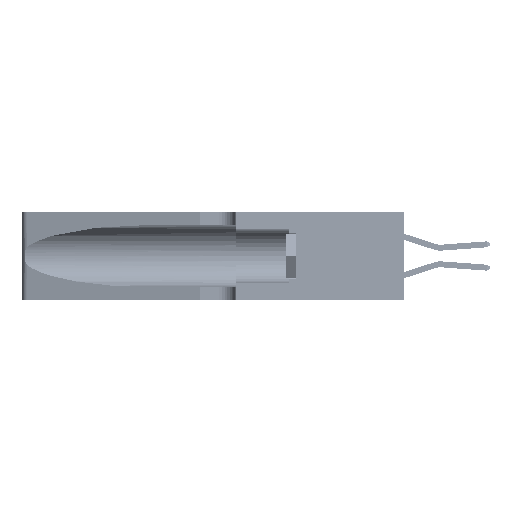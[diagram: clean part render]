
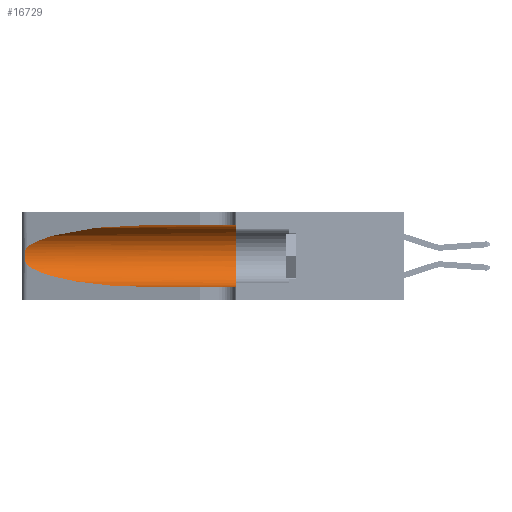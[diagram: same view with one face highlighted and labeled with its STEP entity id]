
A CAD part, left-side view. The second image highlights one B-rep face of the part: STEP entity #16729.
In plain terms, the highlighted cylindrical face has radius 3.308 mm (diameter 6.617 mm), a partial arc.
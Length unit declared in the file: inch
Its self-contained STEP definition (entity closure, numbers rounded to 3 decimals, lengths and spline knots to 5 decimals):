
#296 = CARTESIAN_POINT ( 'NONE',  ( 0.25854, 1.2359, 0.20912 ) ) ;
#1487 = DIRECTION ( 'NONE',  ( 0., -1., 0. ) ) ;
#2696 = FACE_OUTER_BOUND ( 'NONE', #32407, .T. ) ;
#2927 = CARTESIAN_POINT ( 'NONE',  ( 0.1305, 1.61858, 0.185 ) ) ;
#4195 = CARTESIAN_POINT ( 'NONE',  ( 0.1305, 0.35, 0.05475 ) ) ;
#4247 = VECTOR ( 'NONE', #1487, 39.37008 ) ;
#4519 = CARTESIAN_POINT ( 'NONE',  ( 0.25639, 1.23184, 0.21858 ) ) ;
#4634 = CARTESIAN_POINT ( 'NONE',  ( 0.1305, 0.72297, 0.31525 ) ) ;
#5460 = ORIENTED_EDGE ( 'NONE', *, *, #12467, .T. ) ;
#7127 = CARTESIAN_POINT ( 'NONE',  ( 0.25487, 1.22718, 0.14631 ) ) ;
#7469 = CARTESIAN_POINT ( 'NONE',  ( 0.18966, 0.96281, 0.05475 ) ) ;
#8483 = CARTESIAN_POINT ( 'NONE',  ( 0.26075, 1.23896, 0.19203 ) ) ;
#8582 = EDGE_CURVE ( 'NONE', #26187, #10819, #14224, .T. ) ;
#9706 = CARTESIAN_POINT ( 'NONE',  ( 0.25639, 1.23186, 0.15144 ) ) ;
#10405 = CARTESIAN_POINT ( 'NONE',  ( 0.25789, 1.23486, 0.15765 ) ) ;
#10819 = VERTEX_POINT ( 'NONE', #4195 ) ;
#11353 = VERTEX_POINT ( 'NONE', #22461 ) ;
#11595 = DIRECTION ( 'NONE',  ( 0., -1., 0. ) ) ;
#12467 = EDGE_CURVE ( 'NONE', #36347, #12877, #46049, .T. ) ;
#12497 = VERTEX_POINT ( 'NONE', #17984 ) ;
#12662 = CARTESIAN_POINT ( 'NONE',  ( 0.25555, 1.22994, 0.2215 ) ) ;
#12877 = VERTEX_POINT ( 'NONE', #31217 ) ;
#13211 = ORIENTED_EDGE ( 'NONE', *, *, #38663, .T. ) ;
#13757 = EDGE_CURVE ( 'NONE', #12877, #11353, #20491, .T. ) ;
#14224 = LINE ( 'NONE', #40901, #4247 ) ;
#16729 = ADVANCED_FACE ( 'NONE', ( #2696 ), #19548, .F. ) ;
#16826 = CARTESIAN_POINT ( 'NONE',  ( 0.25487, 1.22718, 0.22369 ) ) ;
#17875 = CARTESIAN_POINT ( 'NONE',  ( 0.26075, 1.23896, 0.178 ) ) ;
#17984 = CARTESIAN_POINT ( 'NONE',  ( 0.1305, 0.35, 0.31525 ) ) ;
#19548 = CYLINDRICAL_SURFACE ( 'NONE', #30772, 0.13025 ) ;
#19705 = ORIENTED_EDGE ( 'NONE', *, *, #23955, .F. ) ;
#20341 = CARTESIAN_POINT ( 'NONE',  ( 0.25787, 1.23484, 0.2124 ) ) ;
#20491 = B_SPLINE_CURVE_WITH_KNOTS ( 'NONE', 3,
 ( #16826, #12662, #4519, #20341, #296, #28178, #8483, #17875, #34284, #22074, #10405, #9706, #37609, #45628 ),
 .UNSPECIFIED., .F., .F.,
 ( 4, 2, 2, 2, 2, 2, 4 ),
 ( 0., 0.00027, 0.00053, 0.00107, 0.0016, 0.00187, 0.00214 ),
 .UNSPECIFIED. ) ;
#20998 = ORIENTED_EDGE ( 'NONE', *, *, #13757, .T. ) ;
#22074 = CARTESIAN_POINT ( 'NONE',  ( 0.25856, 1.23593, 0.16098 ) ) ;
#22461 = CARTESIAN_POINT ( 'NONE',  ( 0.25487, 1.22718, 0.14631 ) ) ;
#23955 = EDGE_CURVE ( 'NONE', #36347, #12497, #46667, .T. ) ;
#24228 = DIRECTION ( 'NONE',  ( 0., 1., 0. ) ) ;
#26187 = VERTEX_POINT ( 'NONE', #33351 ) ;
#26600 = DIRECTION ( 'NONE',  ( 0., 0., -1. ) ) ;
#27503 = CARTESIAN_POINT ( 'NONE',  ( 0.1305, 0.72297, 0.05475 ) ) ;
#28178 = CARTESIAN_POINT ( 'NONE',  ( 0.26018, 1.23835, 0.19895 ) ) ;
#29765 =( BOUNDED_CURVE ( )  B_SPLINE_CURVE ( 3, ( #7127, #38864, #7469, #27503 ),
 .UNSPECIFIED., .F., .T. ) 
 B_SPLINE_CURVE_WITH_KNOTS ( ( 4, 4 ),
 ( 3.44316, 4.71239 ),
 .UNSPECIFIED. ) 
 CURVE ( )  GEOMETRIC_REPRESENTATION_ITEM ( )  RATIONAL_B_SPLINE_CURVE ( ( 1., 0.87, 0.87, 1. ) ) 
 REPRESENTATION_ITEM ( '' )  );
#30772 = AXIS2_PLACEMENT_3D ( 'NONE', #2927, #34487, #26600 ) ;
#31217 = CARTESIAN_POINT ( 'NONE',  ( 0.25487, 1.22718, 0.22369 ) ) ;
#31475 = ORIENTED_EDGE ( 'NONE', *, *, #8582, .T. ) ;
#32407 = EDGE_LOOP ( 'NONE', ( #5460, #20998, #13211, #31475, #40556, #19705 ) ) ;
#32592 = DIRECTION ( 'NONE',  ( 0., 0., 1. ) ) ;
#33351 = CARTESIAN_POINT ( 'NONE',  ( 0.1305, 0.72297, 0.05475 ) ) ;
#34284 = CARTESIAN_POINT ( 'NONE',  ( 0.26017, 1.23833, 0.17102 ) ) ;
#34487 = DIRECTION ( 'NONE',  ( 0., -1., 0. ) ) ;
#35540 = AXIS2_PLACEMENT_3D ( 'NONE', #48119, #24228, #32592 ) ;
#36347 = VERTEX_POINT ( 'NONE', #49146 ) ;
#37609 = CARTESIAN_POINT ( 'NONE',  ( 0.25555, 1.22993, 0.14849 ) ) ;
#38663 = EDGE_CURVE ( 'NONE', #11353, #26187, #29765, .T. ) ;
#38864 = CARTESIAN_POINT ( 'NONE',  ( 0.2373, 1.15595, 0.08982 ) ) ;
#40556 = ORIENTED_EDGE ( 'NONE', *, *, #41588, .F. ) ;
#40901 = CARTESIAN_POINT ( 'NONE',  ( 0.1305, 1.61858, 0.05475 ) ) ;
#41098 = VECTOR ( 'NONE', #11595, 39.37008 ) ;
#41588 = EDGE_CURVE ( 'NONE', #12497, #10819, #49746, .T. ) ;
#44874 = CARTESIAN_POINT ( 'NONE',  ( 0.18966, 0.96281, 0.31525 ) ) ;
#45628 = CARTESIAN_POINT ( 'NONE',  ( 0.25487, 1.22718, 0.14631 ) ) ;
#46049 =( BOUNDED_CURVE ( )  B_SPLINE_CURVE ( 3, ( #4634, #44874, #48699, #48524 ),
 .UNSPECIFIED., .F., .F. ) 
 B_SPLINE_CURVE_WITH_KNOTS ( ( 4, 4 ),
 ( 1.5708, 2.84003 ),
 .UNSPECIFIED. ) 
 CURVE ( )  GEOMETRIC_REPRESENTATION_ITEM ( )  RATIONAL_B_SPLINE_CURVE ( ( 1., 0.87, 0.87, 1. ) ) 
 REPRESENTATION_ITEM ( '' )  );
#46619 = CARTESIAN_POINT ( 'NONE',  ( 0.1305, 1.61858, 0.31525 ) ) ;
#46667 = LINE ( 'NONE', #46619, #41098 ) ;
#48119 = CARTESIAN_POINT ( 'NONE',  ( 0.1305, 0.35, 0.185 ) ) ;
#48524 = CARTESIAN_POINT ( 'NONE',  ( 0.25487, 1.22718, 0.22369 ) ) ;
#48699 = CARTESIAN_POINT ( 'NONE',  ( 0.2373, 1.15595, 0.28018 ) ) ;
#49146 = CARTESIAN_POINT ( 'NONE',  ( 0.1305, 0.72297, 0.31525 ) ) ;
#49746 = CIRCLE ( 'NONE', #35540, 0.13025 ) ;
